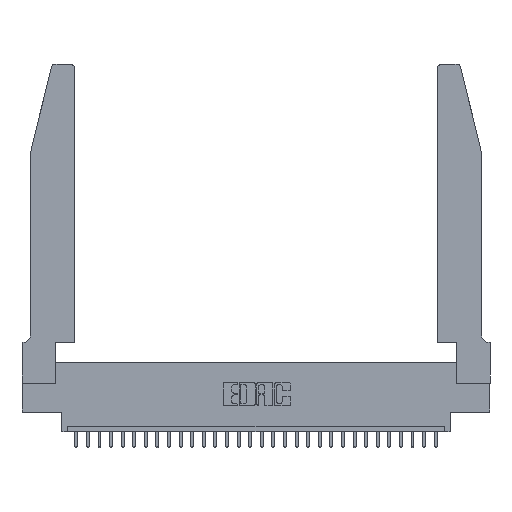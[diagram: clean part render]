
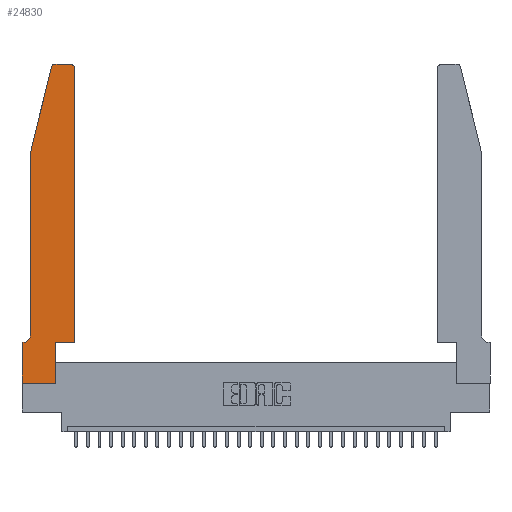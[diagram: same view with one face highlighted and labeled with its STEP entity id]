
A CAD part, top view. The second image highlights one B-rep face of the part: STEP entity #24830.
In plain terms, the highlighted planar face has unit normal (0, 0, 1).
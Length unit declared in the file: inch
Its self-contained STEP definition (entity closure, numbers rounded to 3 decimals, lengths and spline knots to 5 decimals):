
#379 = LINE ( 'NONE', #3581, #30045 ) ;
#515 = VECTOR ( 'NONE', #10830, 39.37008 ) ;
#537 = DIRECTION ( 'NONE',  ( -0.239, -0.971, 0. ) ) ;
#588 = CARTESIAN_POINT ( 'NONE',  ( 0.0755, 0.42, 0.37 ) ) ;
#774 = VERTEX_POINT ( 'NONE', #13062 ) ;
#793 = DIRECTION ( 'NONE',  ( 0., 1., 0. ) ) ;
#895 = LINE ( 'NONE', #15443, #515 ) ;
#1018 = VECTOR ( 'NONE', #29519, 39.37008 ) ;
#1356 = ORIENTED_EDGE ( 'NONE', *, *, #28045, .T. ) ;
#1604 = EDGE_CURVE ( 'NONE', #4473, #10798, #15138, .T. ) ;
#1679 = ORIENTED_EDGE ( 'NONE', *, *, #5132, .T. ) ;
#1938 = CARTESIAN_POINT ( 'NONE',  ( 0.2605, 2.75, 0.37 ) ) ;
#2215 = CARTESIAN_POINT ( 'NONE',  ( 0.284, 2.75, 0.37 ) ) ;
#2319 = DIRECTION ( 'NONE',  ( -1., 0., 0. ) ) ;
#2393 = CARTESIAN_POINT ( 'NONE',  ( 0.4205, 2.75, 0.37 ) ) ;
#2871 = ORIENTED_EDGE ( 'NONE', *, *, #8923, .T. ) ;
#2873 = CARTESIAN_POINT ( 'NONE',  ( 0., 0., 0.37 ) ) ;
#2882 = EDGE_CURVE ( 'NONE', #11832, #4473, #22751, .T. ) ;
#3296 = AXIS2_PLACEMENT_3D ( 'NONE', #4923, #21292, #16700 ) ;
#3581 = CARTESIAN_POINT ( 'NONE',  ( 0., 0., 0.37 ) ) ;
#3871 = DIRECTION ( 'NONE',  ( -1., 0., 0. ) ) ;
#4473 = VERTEX_POINT ( 'NONE', #2393 ) ;
#4923 = CARTESIAN_POINT ( 'NONE',  ( 0.284, 2.72, 0.37 ) ) ;
#5132 = EDGE_CURVE ( 'NONE', #10798, #25843, #28588, .T. ) ;
#5370 = VERTEX_POINT ( 'NONE', #13601 ) ;
#5439 = DIRECTION ( 'NONE',  ( 1., 0., 0. ) ) ;
#5673 = VERTEX_POINT ( 'NONE', #588 ) ;
#6023 = AXIS2_PLACEMENT_3D ( 'NONE', #20851, #6808, #2319 ) ;
#6220 = ORIENTED_EDGE ( 'NONE', *, *, #12735, .T. ) ;
#6569 = VERTEX_POINT ( 'NONE', #13420 ) ;
#6808 = DIRECTION ( 'NONE',  ( 0., 0., -1. ) ) ;
#6831 = ORIENTED_EDGE ( 'NONE', *, *, #12081, .T. ) ;
#8923 = EDGE_CURVE ( 'NONE', #18347, #5370, #16697, .T. ) ;
#9093 = VECTOR ( 'NONE', #3871, 39.37008 ) ;
#9596 = ORIENTED_EDGE ( 'NONE', *, *, #2882, .T. ) ;
#9995 = CARTESIAN_POINT ( 'NONE',  ( 0.0755, 2., 0.37 ) ) ;
#10785 = CARTESIAN_POINT ( 'NONE',  ( 0.2865, 0.35, 0.37 ) ) ;
#10798 = VERTEX_POINT ( 'NONE', #2215 ) ;
#10825 = ORIENTED_EDGE ( 'NONE', *, *, #29032, .T. ) ;
#10830 = DIRECTION ( 'NONE',  ( 1., 0., 0. ) ) ;
#11003 = LINE ( 'NONE', #23127, #28191 ) ;
#11519 = VERTEX_POINT ( 'NONE', #27298 ) ;
#11832 = VERTEX_POINT ( 'NONE', #25735 ) ;
#12081 = EDGE_CURVE ( 'NONE', #12676, #18347, #28875, .T. ) ;
#12502 = CARTESIAN_POINT ( 'NONE',  ( 0., 0.35, 0.37 ) ) ;
#12676 = VERTEX_POINT ( 'NONE', #2873 ) ;
#12735 = EDGE_CURVE ( 'NONE', #774, #11519, #17184, .T. ) ;
#13062 = CARTESIAN_POINT ( 'NONE',  ( 0.0055, 0.35, 0.37 ) ) ;
#13420 = CARTESIAN_POINT ( 'NONE',  ( 0.4505, 0.35, 0.37 ) ) ;
#13601 = CARTESIAN_POINT ( 'NONE',  ( 0.2865, 0.35, 0.37 ) ) ;
#13785 = FACE_OUTER_BOUND ( 'NONE', #22132, .T. ) ;
#14487 = VECTOR ( 'NONE', #24894, 39.37008 ) ;
#14536 = VERTEX_POINT ( 'NONE', #26896 ) ;
#14660 = DIRECTION ( 'NONE',  ( 0., 0., 1. ) ) ;
#14736 = EDGE_CURVE ( 'NONE', #5673, #774, #15953, .T. ) ;
#14824 = ORIENTED_EDGE ( 'NONE', *, *, #17194, .T. ) ;
#15138 = LINE ( 'NONE', #1938, #21721 ) ;
#15443 = CARTESIAN_POINT ( 'NONE',  ( 0.4505, 0.35, 0.37 ) ) ;
#15699 = CARTESIAN_POINT ( 'NONE',  ( 0.2865, 0., 0.37 ) ) ;
#15953 = CIRCLE ( 'NONE', #6023, 0.07 ) ;
#16065 = ORIENTED_EDGE ( 'NONE', *, *, #14736, .T. ) ;
#16697 = LINE ( 'NONE', #10785, #14487 ) ;
#16700 = DIRECTION ( 'NONE',  ( 1., 0., 0. ) ) ;
#17127 = LINE ( 'NONE', #22026, #28082 ) ;
#17184 = LINE ( 'NONE', #27388, #9093 ) ;
#17194 = EDGE_CURVE ( 'NONE', #14536, #5673, #11003, .T. ) ;
#18236 = DIRECTION ( 'NONE',  ( 0., -1., 0. ) ) ;
#18347 = VERTEX_POINT ( 'NONE', #15699 ) ;
#18446 = ORIENTED_EDGE ( 'NONE', *, *, #1604, .T. ) ;
#20269 = DIRECTION ( 'NONE',  ( 0., 0., 1. ) ) ;
#20851 = CARTESIAN_POINT ( 'NONE',  ( 0.0055, 0.42, 0.37 ) ) ;
#21292 = DIRECTION ( 'NONE',  ( 0., 0., 1. ) ) ;
#21527 = EDGE_CURVE ( 'NONE', #5370, #6569, #895, .T. ) ;
#21721 = VECTOR ( 'NONE', #25373, 39.37008 ) ;
#21889 = AXIS2_PLACEMENT_3D ( 'NONE', #12502, #14660, #5439 ) ;
#21912 = ORIENTED_EDGE ( 'NONE', *, *, #21527, .T. ) ;
#22026 = CARTESIAN_POINT ( 'NONE',  ( 0.4505, 0.35, 0.37 ) ) ;
#22132 = EDGE_LOOP ( 'NONE', ( #18446, #1679, #10825, #14824, #16065, #6220, #1356, #6831, #2871, #21912, #28475, #9596 ) ) ;
#22318 = DIRECTION ( 'NONE',  ( 0., -1., 0. ) ) ;
#22330 = LINE ( 'NONE', #9995, #28138 ) ;
#22751 = CIRCLE ( 'NONE', #23650, 0.03 ) ;
#22930 = DIRECTION ( 'NONE',  ( 1., 0., 0. ) ) ;
#23127 = CARTESIAN_POINT ( 'NONE',  ( 0.0755, 2., 0.37 ) ) ;
#23650 = AXIS2_PLACEMENT_3D ( 'NONE', #25156, #20269, #22930 ) ;
#24169 = PLANE ( 'NONE',  #21889 ) ;
#24830 = ADVANCED_FACE ( 'NONE', ( #13785 ), #24169, .T. ) ;
#24894 = DIRECTION ( 'NONE',  ( 0., 1., 0. ) ) ;
#25156 = CARTESIAN_POINT ( 'NONE',  ( 0.4205, 2.72, 0.37 ) ) ;
#25373 = DIRECTION ( 'NONE',  ( -1., 0., 0. ) ) ;
#25735 = CARTESIAN_POINT ( 'NONE',  ( 0.4505, 2.72, 0.37 ) ) ;
#25843 = VERTEX_POINT ( 'NONE', #28399 ) ;
#26584 = CARTESIAN_POINT ( 'NONE',  ( 0., 0., 0.37 ) ) ;
#26896 = CARTESIAN_POINT ( 'NONE',  ( 0.0755, 2., 0.37 ) ) ;
#27298 = CARTESIAN_POINT ( 'NONE',  ( 0., 0.35, 0.37 ) ) ;
#27388 = CARTESIAN_POINT ( 'NONE',  ( 0.0755, 0.35, 0.37 ) ) ;
#28045 = EDGE_CURVE ( 'NONE', #11519, #12676, #379, .T. ) ;
#28082 = VECTOR ( 'NONE', #793, 39.37008 ) ;
#28138 = VECTOR ( 'NONE', #537, 39.37008 ) ;
#28191 = VECTOR ( 'NONE', #18236, 39.37008 ) ;
#28399 = CARTESIAN_POINT ( 'NONE',  ( 0.25487, 2.72718, 0.37 ) ) ;
#28475 = ORIENTED_EDGE ( 'NONE', *, *, #29831, .T. ) ;
#28588 = CIRCLE ( 'NONE', #3296, 0.03 ) ;
#28875 = LINE ( 'NONE', #26584, #1018 ) ;
#29032 = EDGE_CURVE ( 'NONE', #25843, #14536, #22330, .T. ) ;
#29519 = DIRECTION ( 'NONE',  ( 1., 0., 0. ) ) ;
#29831 = EDGE_CURVE ( 'NONE', #6569, #11832, #17127, .T. ) ;
#30045 = VECTOR ( 'NONE', #22318, 39.37008 ) ;
